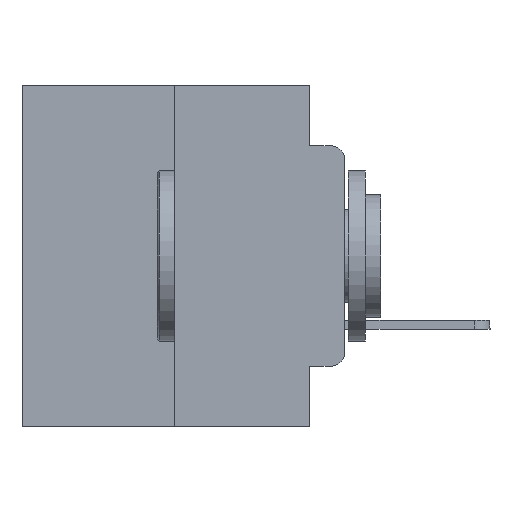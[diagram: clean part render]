
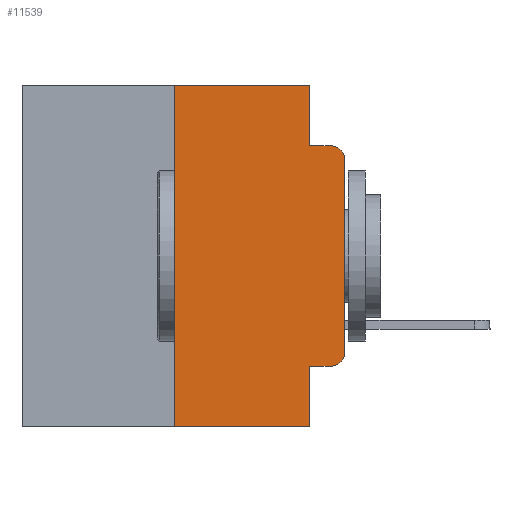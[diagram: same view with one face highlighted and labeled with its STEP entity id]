
A CAD part, left-side view. The second image highlights one B-rep face of the part: STEP entity #11539.
In plain terms, the highlighted planar face has unit normal (-1, 0, 0).
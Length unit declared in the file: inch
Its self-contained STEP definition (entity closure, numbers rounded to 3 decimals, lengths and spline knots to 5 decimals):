
#368 = DIRECTION ( 'NONE',  ( -1., 0., 0. ) ) ;
#611 = EDGE_CURVE ( 'NONE', #7234, #17387, #12742, .T. ) ;
#646 = DIRECTION ( 'NONE',  ( 0., -1., 0. ) ) ;
#961 = DIRECTION ( 'NONE',  ( -1., 0., 0. ) ) ;
#1189 = AXIS2_PLACEMENT_3D ( 'NONE', #9450, #17950, #5391 ) ;
#1522 = VERTEX_POINT ( 'NONE', #9581 ) ;
#2328 = VERTEX_POINT ( 'NONE', #13992 ) ;
#2432 = DIRECTION ( 'NONE',  ( 0., -1., 0. ) ) ;
#2462 = CARTESIAN_POINT ( 'NONE',  ( 0., 0.02, -0.3915 ) ) ;
#2872 = VECTOR ( 'NONE', #9657, 39.37008 ) ;
#3217 = EDGE_CURVE ( 'NONE', #19384, #20793, #9711, .T. ) ;
#3652 = VECTOR ( 'NONE', #646, 39.37008 ) ;
#4282 = AXIS2_PLACEMENT_3D ( 'NONE', #2462, #368, #8862 ) ;
#4861 = CARTESIAN_POINT ( 'NONE',  ( 0., 0., 0. ) ) ;
#5391 = DIRECTION ( 'NONE',  ( 0., 0., -1. ) ) ;
#5931 = CARTESIAN_POINT ( 'NONE',  ( 0., 0.02, -0.0885 ) ) ;
#6214 = LINE ( 'NONE', #14722, #23085 ) ;
#6348 = EDGE_CURVE ( 'NONE', #7639, #2328, #26498, .T. ) ;
#6471 = VERTEX_POINT ( 'NONE', #27201 ) ;
#6825 = DIRECTION ( 'NONE',  ( 0., -1., 0. ) ) ;
#7114 = ORIENTED_EDGE ( 'NONE', *, *, #3217, .F. ) ;
#7234 = VERTEX_POINT ( 'NONE', #8175 ) ;
#7490 = PLANE ( 'NONE',  #1189 ) ;
#7639 = VERTEX_POINT ( 'NONE', #10375 ) ;
#8175 = CARTESIAN_POINT ( 'NONE',  ( 0., 0.02, -0.4115 ) ) ;
#8289 = CARTESIAN_POINT ( 'NONE',  ( 0., 0., -0.3915 ) ) ;
#8463 = ORIENTED_EDGE ( 'NONE', *, *, #20170, .T. ) ;
#8559 = LINE ( 'NONE', #23180, #17773 ) ;
#8640 = EDGE_LOOP ( 'NONE', ( #8463, #20036, #7114, #18708, #13574, #14514, #25484, #16821, #26756, #18000 ) ) ;
#8664 = EDGE_CURVE ( 'NONE', #2328, #16812, #19706, .T. ) ;
#8862 = DIRECTION ( 'NONE',  ( 0., 0., -1. ) ) ;
#9450 = CARTESIAN_POINT ( 'NONE',  ( 0., 0.473, 0. ) ) ;
#9581 = CARTESIAN_POINT ( 'NONE',  ( 0., 0., -0.1085 ) ) ;
#9657 = DIRECTION ( 'NONE',  ( 0., 0., 1. ) ) ;
#9711 = LINE ( 'NONE', #26970, #27186 ) ;
#9718 = DIRECTION ( 'NONE',  ( 0., 0., -1. ) ) ;
#10375 = CARTESIAN_POINT ( 'NONE',  ( 0., 0.25, -0.5 ) ) ;
#10457 = EDGE_CURVE ( 'NONE', #7639, #6471, #8559, .T. ) ;
#10990 = EDGE_CURVE ( 'NONE', #23147, #7234, #25909, .T. ) ;
#11278 = LINE ( 'NONE', #4861, #11978 ) ;
#11421 = CARTESIAN_POINT ( 'NONE',  ( 0., 0.051, -0.4115 ) ) ;
#11467 = EDGE_CURVE ( 'NONE', #1522, #20793, #13849, .T. ) ;
#11539 = ADVANCED_FACE ( 'NONE', ( #16268 ), #7490, .F. ) ;
#11616 = AXIS2_PLACEMENT_3D ( 'NONE', #18379, #961, #9718 ) ;
#11705 = EDGE_CURVE ( 'NONE', #23147, #6471, #6214, .T. ) ;
#11978 = VECTOR ( 'NONE', #23809, 39.37008 ) ;
#12742 = CIRCLE ( 'NONE', #4282, 0.02 ) ;
#12746 = DIRECTION ( 'NONE',  ( 0., 0., -1. ) ) ;
#13574 = ORIENTED_EDGE ( 'NONE', *, *, #8664, .F. ) ;
#13849 = CIRCLE ( 'NONE', #11616, 0.02 ) ;
#13992 = CARTESIAN_POINT ( 'NONE',  ( 0., 0.25, 0. ) ) ;
#14514 = ORIENTED_EDGE ( 'NONE', *, *, #6348, .F. ) ;
#14722 = CARTESIAN_POINT ( 'NONE',  ( 0., 0.051, 0. ) ) ;
#14959 = LINE ( 'NONE', #17210, #24824 ) ;
#15937 = CARTESIAN_POINT ( 'NONE',  ( 0., 0.25, 0. ) ) ;
#16268 = FACE_OUTER_BOUND ( 'NONE', #8640, .T. ) ;
#16812 = VERTEX_POINT ( 'NONE', #18374 ) ;
#16821 = ORIENTED_EDGE ( 'NONE', *, *, #11705, .F. ) ;
#17085 = CARTESIAN_POINT ( 'NONE',  ( 0., 0.473, 0. ) ) ;
#17210 = CARTESIAN_POINT ( 'NONE',  ( 0., 0.051, 0. ) ) ;
#17387 = VERTEX_POINT ( 'NONE', #8289 ) ;
#17773 = VECTOR ( 'NONE', #2432, 39.37008 ) ;
#17950 = DIRECTION ( 'NONE',  ( 1., 0., 0. ) ) ;
#18000 = ORIENTED_EDGE ( 'NONE', *, *, #611, .T. ) ;
#18374 = CARTESIAN_POINT ( 'NONE',  ( 0., 0.051, 0. ) ) ;
#18379 = CARTESIAN_POINT ( 'NONE',  ( 0., 0.02, -0.1085 ) ) ;
#18465 = CARTESIAN_POINT ( 'NONE',  ( 0., 0.051, -0.0885 ) ) ;
#18708 = ORIENTED_EDGE ( 'NONE', *, *, #19090, .F. ) ;
#19090 = EDGE_CURVE ( 'NONE', #16812, #19384, #14959, .T. ) ;
#19384 = VERTEX_POINT ( 'NONE', #18465 ) ;
#19706 = LINE ( 'NONE', #17085, #3652 ) ;
#20036 = ORIENTED_EDGE ( 'NONE', *, *, #11467, .T. ) ;
#20170 = EDGE_CURVE ( 'NONE', #17387, #1522, #11278, .T. ) ;
#20793 = VERTEX_POINT ( 'NONE', #5931 ) ;
#21463 = CARTESIAN_POINT ( 'NONE',  ( 0., 0.051, -0.4115 ) ) ;
#23085 = VECTOR ( 'NONE', #23222, 39.37008 ) ;
#23147 = VERTEX_POINT ( 'NONE', #21463 ) ;
#23180 = CARTESIAN_POINT ( 'NONE',  ( 0., 0.473, -0.5 ) ) ;
#23222 = DIRECTION ( 'NONE',  ( 0., 0., -1. ) ) ;
#23809 = DIRECTION ( 'NONE',  ( 0., 0., 1. ) ) ;
#24824 = VECTOR ( 'NONE', #12746, 39.37008 ) ;
#25484 = ORIENTED_EDGE ( 'NONE', *, *, #10457, .T. ) ;
#25909 = LINE ( 'NONE', #11421, #27259 ) ;
#26498 = LINE ( 'NONE', #15937, #2872 ) ;
#26690 = DIRECTION ( 'NONE',  ( 0., -1., 0. ) ) ;
#26756 = ORIENTED_EDGE ( 'NONE', *, *, #10990, .T. ) ;
#26970 = CARTESIAN_POINT ( 'NONE',  ( 0., 0.051, -0.0885 ) ) ;
#27186 = VECTOR ( 'NONE', #26690, 39.37008 ) ;
#27201 = CARTESIAN_POINT ( 'NONE',  ( 0., 0.051, -0.5 ) ) ;
#27259 = VECTOR ( 'NONE', #6825, 39.37008 ) ;
